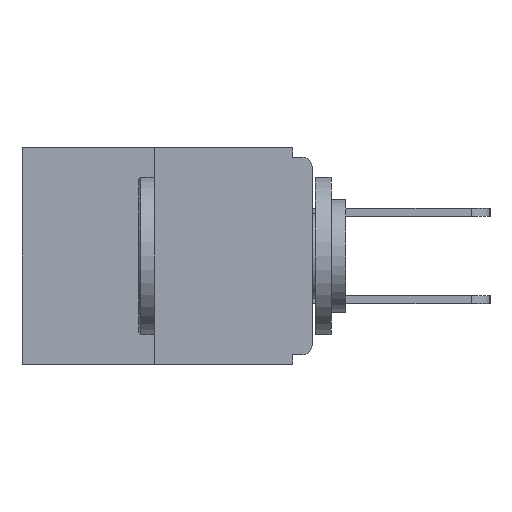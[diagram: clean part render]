
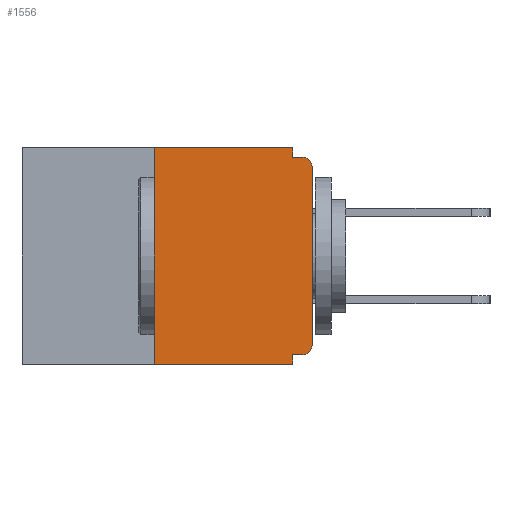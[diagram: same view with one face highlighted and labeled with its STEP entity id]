
A CAD part, left-side view. The second image highlights one B-rep face of the part: STEP entity #1556.
In plain terms, the highlighted planar face has unit normal (-1, 0, 0).
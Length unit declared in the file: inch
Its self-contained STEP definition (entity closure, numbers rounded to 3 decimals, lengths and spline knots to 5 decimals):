
#138 = LINE ( 'NONE', #14507, #7146 ) ;
#259 = LINE ( 'NONE', #18061, #2821 ) ;
#268 = CARTESIAN_POINT ( 'NONE',  ( 0., 0.015, -0.03 ) ) ;
#443 = ORIENTED_EDGE ( 'NONE', *, *, #9614, .T. ) ;
#456 = CARTESIAN_POINT ( 'NONE',  ( 0., 0.015, -0.328 ) ) ;
#878 = CARTESIAN_POINT ( 'NONE',  ( 0., 0.46, -0.343 ) ) ;
#1081 = VERTEX_POINT ( 'NONE', #19919 ) ;
#1142 = AXIS2_PLACEMENT_3D ( 'NONE', #18411, #3897, #6227 ) ;
#1556 = ADVANCED_FACE ( 'NONE', ( #18406 ), #6087, .F. ) ;
#2099 = VECTOR ( 'NONE', #13064, 39.37008 ) ;
#2821 = VECTOR ( 'NONE', #6130, 39.37008 ) ;
#3470 = VERTEX_POINT ( 'NONE', #10412 ) ;
#3897 = DIRECTION ( 'NONE',  ( -1., 0., 0. ) ) ;
#4025 = VERTEX_POINT ( 'NONE', #6269 ) ;
#4405 = CARTESIAN_POINT ( 'NONE',  ( 0., 0.031, -0.328 ) ) ;
#4487 = ORIENTED_EDGE ( 'NONE', *, *, #15633, .F. ) ;
#4655 = LINE ( 'NONE', #11007, #2099 ) ;
#4910 = VECTOR ( 'NONE', #9023, 39.37008 ) ;
#5072 = EDGE_CURVE ( 'NONE', #21502, #9204, #23025, .T. ) ;
#6087 = PLANE ( 'NONE',  #24688 ) ;
#6130 = DIRECTION ( 'NONE',  ( 0., -1., 0. ) ) ;
#6185 = CARTESIAN_POINT ( 'NONE',  ( 0., 0.25, -0.343 ) ) ;
#6227 = DIRECTION ( 'NONE',  ( 0., 0., -1. ) ) ;
#6269 = CARTESIAN_POINT ( 'NONE',  ( 0., 0.031, -0.015 ) ) ;
#6912 = ORIENTED_EDGE ( 'NONE', *, *, #23101, .F. ) ;
#7146 = VECTOR ( 'NONE', #16523, 39.37008 ) ;
#7501 = CARTESIAN_POINT ( 'NONE',  ( 0., 0.015, -0.015 ) ) ;
#7582 = LINE ( 'NONE', #25292, #8221 ) ;
#8087 = EDGE_CURVE ( 'NONE', #22544, #1081, #259, .T. ) ;
#8221 = VECTOR ( 'NONE', #19382, 39.37008 ) ;
#8636 = ORIENTED_EDGE ( 'NONE', *, *, #24219, .T. ) ;
#8662 = DIRECTION ( 'NONE',  ( 0., 1., 0. ) ) ;
#9023 = DIRECTION ( 'NONE',  ( 0., 0., 1. ) ) ;
#9204 = VERTEX_POINT ( 'NONE', #7501 ) ;
#9614 = EDGE_CURVE ( 'NONE', #15752, #12535, #12367, .T. ) ;
#9634 = CARTESIAN_POINT ( 'NONE',  ( 0., 0.031, 0. ) ) ;
#10412 = CARTESIAN_POINT ( 'NONE',  ( 0., 0., -0.313 ) ) ;
#10722 = ORIENTED_EDGE ( 'NONE', *, *, #8087, .F. ) ;
#10761 = CARTESIAN_POINT ( 'NONE',  ( 0., 0., -0.328 ) ) ;
#11007 = CARTESIAN_POINT ( 'NONE',  ( 0., 0., 0. ) ) ;
#11853 = VERTEX_POINT ( 'NONE', #456 ) ;
#11981 = CARTESIAN_POINT ( 'NONE',  ( 0., 0.46, 0. ) ) ;
#12367 = LINE ( 'NONE', #878, #25084 ) ;
#12535 = VERTEX_POINT ( 'NONE', #23665 ) ;
#12927 = ORIENTED_EDGE ( 'NONE', *, *, #20179, .F. ) ;
#13064 = DIRECTION ( 'NONE',  ( 0., 0., 1. ) ) ;
#14507 = CARTESIAN_POINT ( 'NONE',  ( 0., 0., -0.015 ) ) ;
#14771 = EDGE_CURVE ( 'NONE', #3470, #21502, #4655, .T. ) ;
#15093 = LINE ( 'NONE', #9634, #18879 ) ;
#15545 = EDGE_CURVE ( 'NONE', #4025, #9204, #138, .T. ) ;
#15633 = EDGE_CURVE ( 'NONE', #15752, #22544, #18600, .T. ) ;
#15704 = DIRECTION ( 'NONE',  ( 0., 0., -1. ) ) ;
#15752 = VERTEX_POINT ( 'NONE', #6185 ) ;
#16010 = ORIENTED_EDGE ( 'NONE', *, *, #23818, .F. ) ;
#16055 = VECTOR ( 'NONE', #8662, 39.37008 ) ;
#16523 = DIRECTION ( 'NONE',  ( 0., -1., 0. ) ) ;
#16554 = DIRECTION ( 'NONE',  ( -1., 0., 0. ) ) ;
#17439 = VERTEX_POINT ( 'NONE', #4405 ) ;
#18061 = CARTESIAN_POINT ( 'NONE',  ( 0., 0.46, 0. ) ) ;
#18105 = DIRECTION ( 'NONE',  ( 0., 0., -1. ) ) ;
#18406 = FACE_OUTER_BOUND ( 'NONE', #22355, .T. ) ;
#18411 = CARTESIAN_POINT ( 'NONE',  ( 0., 0.015, -0.313 ) ) ;
#18600 = LINE ( 'NONE', #25083, #4910 ) ;
#18879 = VECTOR ( 'NONE', #15704, 39.37008 ) ;
#18989 = ORIENTED_EDGE ( 'NONE', *, *, #5072, .T. ) ;
#19382 = DIRECTION ( 'NONE',  ( 0., 0., -1. ) ) ;
#19919 = CARTESIAN_POINT ( 'NONE',  ( 0., 0.031, 0. ) ) ;
#20179 = EDGE_CURVE ( 'NONE', #17439, #12535, #7582, .T. ) ;
#21441 = LINE ( 'NONE', #10761, #16055 ) ;
#21502 = VERTEX_POINT ( 'NONE', #21578 ) ;
#21578 = CARTESIAN_POINT ( 'NONE',  ( 0., 0., -0.03 ) ) ;
#22165 = DIRECTION ( 'NONE',  ( 1., 0., 0. ) ) ;
#22355 = EDGE_LOOP ( 'NONE', ( #10722, #4487, #443, #12927, #6912, #8636, #25233, #18989, #22716, #16010 ) ) ;
#22544 = VERTEX_POINT ( 'NONE', #23049 ) ;
#22680 = DIRECTION ( 'NONE',  ( 0., 0., -1. ) ) ;
#22716 = ORIENTED_EDGE ( 'NONE', *, *, #15545, .F. ) ;
#22860 = DIRECTION ( 'NONE',  ( 0., -1., 0. ) ) ;
#23025 = CIRCLE ( 'NONE', #26276, 0.015 ) ;
#23049 = CARTESIAN_POINT ( 'NONE',  ( 0., 0.25, 0. ) ) ;
#23101 = EDGE_CURVE ( 'NONE', #11853, #17439, #21441, .T. ) ;
#23665 = CARTESIAN_POINT ( 'NONE',  ( 0., 0.031, -0.343 ) ) ;
#23818 = EDGE_CURVE ( 'NONE', #1081, #4025, #15093, .T. ) ;
#24219 = EDGE_CURVE ( 'NONE', #11853, #3470, #24581, .T. ) ;
#24581 = CIRCLE ( 'NONE', #1142, 0.015 ) ;
#24688 = AXIS2_PLACEMENT_3D ( 'NONE', #11981, #22165, #18105 ) ;
#25083 = CARTESIAN_POINT ( 'NONE',  ( 0., 0.25, 0. ) ) ;
#25084 = VECTOR ( 'NONE', #22860, 39.37008 ) ;
#25233 = ORIENTED_EDGE ( 'NONE', *, *, #14771, .T. ) ;
#25292 = CARTESIAN_POINT ( 'NONE',  ( 0., 0.031, -0.343 ) ) ;
#26276 = AXIS2_PLACEMENT_3D ( 'NONE', #268, #16554, #22680 ) ;
